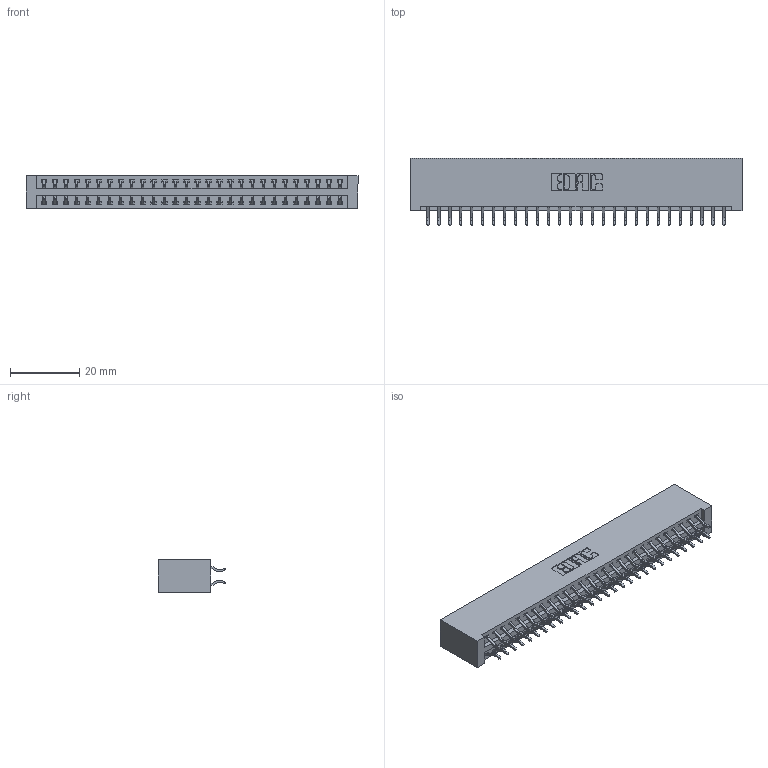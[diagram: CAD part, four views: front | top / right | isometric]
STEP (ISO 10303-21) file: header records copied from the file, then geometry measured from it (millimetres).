
FILE_DESCRIPTION (( 'STEP AP203' ), '1' );
FILE_NAME ('346-056-556-201.STEP', '2018-08-28T03:03:14', ( '' ), ( '' ), 'SwSTEP 2.0', 'SolidWorks 2016', '' );
FILE_SCHEMA (( 'CONFIG_CONTROL_DESIGN' ));
Length unit declared in the file: inch
Products named in the file (3): 346 Part_No Mounting Lugs; 345-292-001_556 Tail; 346-056-556-201
Assembly tree (57 placements, depth 2):
  346-056-556-201
    346 Part_No Mounting Lugs
    345-292-001_556 Tail  x56
Bounding box: 96.14 x 19.57 x 9.4 mm (x, y, z)
Volume: 9837.1 mm3; surface area: 13412.8 mm2
Topology: 57 solids, 57 shells, 3362 faces, 9993 edges, 6586 vertices
Faces by surface type: plane 2256, cylinder 1106
Entity records: 20101 total; most frequent: CARTESIAN_POINT 3344, ORIENTED_EDGE 3266, DIRECTION 2981, EDGE_CURVE 1633, LINE 1389, VECTOR 1389, VERTEX_POINT 1086, AXIS2_PLACEMENT_3D 796
